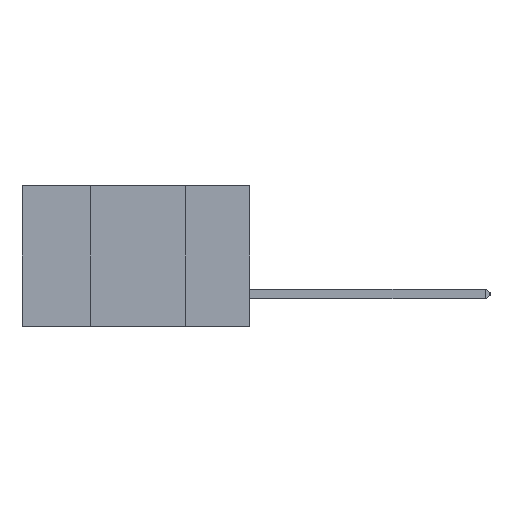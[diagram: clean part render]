
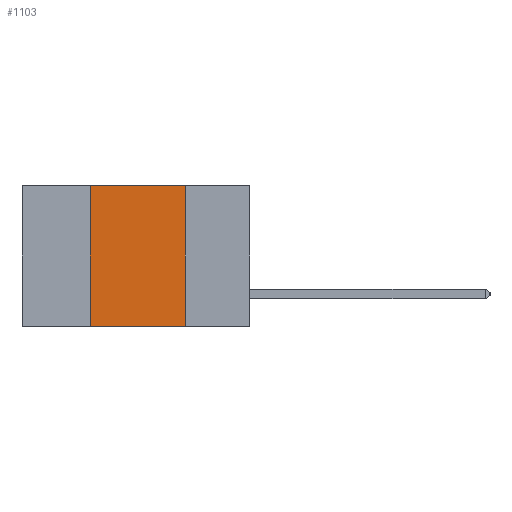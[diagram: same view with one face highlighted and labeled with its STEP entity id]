
A CAD part, left-side view. The second image highlights one B-rep face of the part: STEP entity #1103.
In plain terms, the highlighted planar face has unit normal (-1, 0, 0).
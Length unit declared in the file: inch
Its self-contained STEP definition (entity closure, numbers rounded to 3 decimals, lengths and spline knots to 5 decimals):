
#299 = CARTESIAN_POINT ( 'NONE',  ( 0., 0.17, -0.37 ) ) ;
#1103 = ADVANCED_FACE ( 'NONE', ( #16767 ), #1105, .F. ) ;
#1105 = PLANE ( 'NONE',  #2060 ) ;
#1580 = DIRECTION ( 'NONE',  ( 0., 0., 1. ) ) ;
#1650 = LINE ( 'NONE', #18754, #21409 ) ;
#2060 = AXIS2_PLACEMENT_3D ( 'NONE', #14595, #13123, #14828 ) ;
#2669 = VECTOR ( 'NONE', #13606, 39.37008 ) ;
#5673 = VERTEX_POINT ( 'NONE', #19540 ) ;
#5831 = CARTESIAN_POINT ( 'NONE',  ( 0., 0.17, 0. ) ) ;
#6171 = ORIENTED_EDGE ( 'NONE', *, *, #16670, .F. ) ;
#6887 = VERTEX_POINT ( 'NONE', #5831 ) ;
#8430 = CARTESIAN_POINT ( 'NONE',  ( 0., 0.42, 0. ) ) ;
#8487 = LINE ( 'NONE', #18399, #2669 ) ;
#9461 = VERTEX_POINT ( 'NONE', #299 ) ;
#9494 = VECTOR ( 'NONE', #1580, 39.37008 ) ;
#10041 = EDGE_CURVE ( 'NONE', #21325, #9461, #20875, .T. ) ;
#11775 = CARTESIAN_POINT ( 'NONE',  ( 0., 0.42, -0.37 ) ) ;
#11988 = DIRECTION ( 'NONE',  ( 0., -1., 0. ) ) ;
#12108 = ORIENTED_EDGE ( 'NONE', *, *, #14571, .F. ) ;
#12987 = EDGE_LOOP ( 'NONE', ( #14873, #12108, #6171, #21692 ) ) ;
#13123 = DIRECTION ( 'NONE',  ( 1., 0., 0. ) ) ;
#13606 = DIRECTION ( 'NONE',  ( 0., 0., -1. ) ) ;
#14571 = EDGE_CURVE ( 'NONE', #5673, #6887, #1650, .T. ) ;
#14595 = CARTESIAN_POINT ( 'NONE',  ( 0., 0.6, 0. ) ) ;
#14745 = LINE ( 'NONE', #8430, #9494 ) ;
#14828 = DIRECTION ( 'NONE',  ( 0., 0., -1. ) ) ;
#14873 = ORIENTED_EDGE ( 'NONE', *, *, #20030, .F. ) ;
#16454 = VECTOR ( 'NONE', #18023, 39.37008 ) ;
#16670 = EDGE_CURVE ( 'NONE', #21325, #5673, #14745, .T. ) ;
#16767 = FACE_OUTER_BOUND ( 'NONE', #12987, .T. ) ;
#18023 = DIRECTION ( 'NONE',  ( 0., -1., 0. ) ) ;
#18399 = CARTESIAN_POINT ( 'NONE',  ( 0., 0.17, 0. ) ) ;
#18754 = CARTESIAN_POINT ( 'NONE',  ( 0., 0.6, 0. ) ) ;
#19412 = CARTESIAN_POINT ( 'NONE',  ( 0., 0.6, -0.37 ) ) ;
#19540 = CARTESIAN_POINT ( 'NONE',  ( 0., 0.42, 0. ) ) ;
#20030 = EDGE_CURVE ( 'NONE', #6887, #9461, #8487, .T. ) ;
#20875 = LINE ( 'NONE', #19412, #16454 ) ;
#21325 = VERTEX_POINT ( 'NONE', #11775 ) ;
#21409 = VECTOR ( 'NONE', #11988, 39.37008 ) ;
#21692 = ORIENTED_EDGE ( 'NONE', *, *, #10041, .T. ) ;
